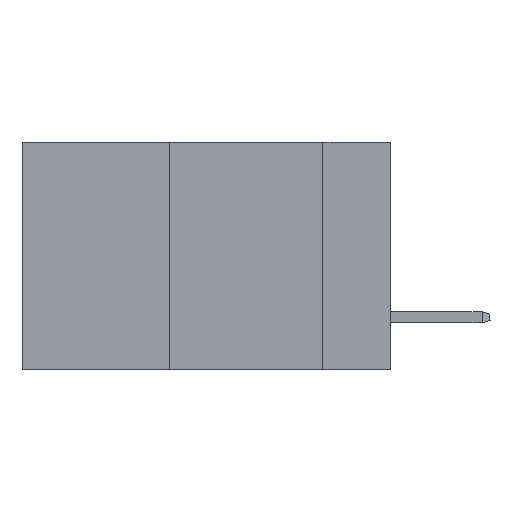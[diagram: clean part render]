
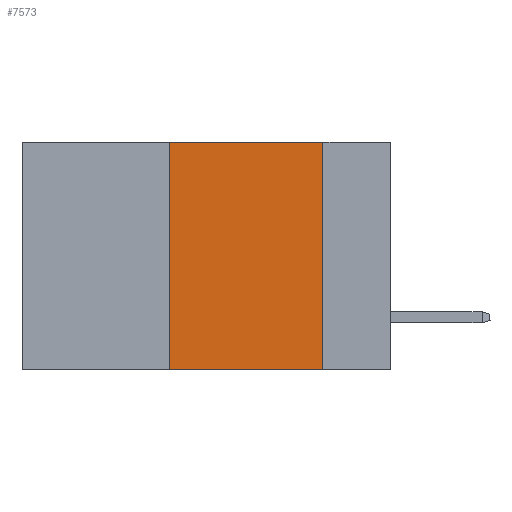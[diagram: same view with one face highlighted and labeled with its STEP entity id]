
A CAD part, left-side view. The second image highlights one B-rep face of the part: STEP entity #7573.
In plain terms, the highlighted planar face has unit normal (-1, 0, 0).
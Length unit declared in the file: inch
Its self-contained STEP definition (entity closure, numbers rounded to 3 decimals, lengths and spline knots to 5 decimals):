
#1581 = VERTEX_POINT ( 'NONE', #14168 ) ;
#2299 = CARTESIAN_POINT ( 'NONE',  ( 0., 0.6, 0. ) ) ;
#2630 = DIRECTION ( 'NONE',  ( 0., 0., 1. ) ) ;
#3294 = VECTOR ( 'NONE', #2630, 39.37008 ) ;
#3382 = CARTESIAN_POINT ( 'NONE',  ( 0., 0.36, -0.37 ) ) ;
#4561 = ORIENTED_EDGE ( 'NONE', *, *, #7499, .F. ) ;
#5371 = CARTESIAN_POINT ( 'NONE',  ( 0., 0.11, 0. ) ) ;
#6660 = EDGE_CURVE ( 'NONE', #1581, #9404, #7897, .T. ) ;
#7148 = ORIENTED_EDGE ( 'NONE', *, *, #10180, .F. ) ;
#7499 = EDGE_CURVE ( 'NONE', #10440, #1581, #23999, .T. ) ;
#7573 = ADVANCED_FACE ( 'NONE', ( #11313 ), #7975, .F. ) ;
#7605 = CARTESIAN_POINT ( 'NONE',  ( 0., 0.11, -0.37 ) ) ;
#7897 = LINE ( 'NONE', #5371, #25316 ) ;
#7975 = PLANE ( 'NONE',  #8375 ) ;
#8375 = AXIS2_PLACEMENT_3D ( 'NONE', #22219, #16552, #22559 ) ;
#8547 = EDGE_LOOP ( 'NONE', ( #12255, #4561, #7148, #10906 ) ) ;
#8952 = CARTESIAN_POINT ( 'NONE',  ( 0., 0.6, -0.37 ) ) ;
#9338 = CARTESIAN_POINT ( 'NONE',  ( 0., 0.36, 0. ) ) ;
#9404 = VERTEX_POINT ( 'NONE', #7605 ) ;
#10180 = EDGE_CURVE ( 'NONE', #14652, #10440, #14028, .T. ) ;
#10440 = VERTEX_POINT ( 'NONE', #9338 ) ;
#10906 = ORIENTED_EDGE ( 'NONE', *, *, #21439, .T. ) ;
#11313 = FACE_OUTER_BOUND ( 'NONE', #8547, .T. ) ;
#12255 = ORIENTED_EDGE ( 'NONE', *, *, #6660, .F. ) ;
#14028 = LINE ( 'NONE', #23514, #3294 ) ;
#14168 = CARTESIAN_POINT ( 'NONE',  ( 0., 0.11, 0. ) ) ;
#14652 = VERTEX_POINT ( 'NONE', #3382 ) ;
#15391 = LINE ( 'NONE', #8952, #19864 ) ;
#15756 = DIRECTION ( 'NONE',  ( 0., -1., 0. ) ) ;
#16365 = VECTOR ( 'NONE', #16475, 39.37008 ) ;
#16475 = DIRECTION ( 'NONE',  ( 0., -1., 0. ) ) ;
#16552 = DIRECTION ( 'NONE',  ( 1., 0., 0. ) ) ;
#19864 = VECTOR ( 'NONE', #15756, 39.37008 ) ;
#21439 = EDGE_CURVE ( 'NONE', #14652, #9404, #15391, .T. ) ;
#21597 = DIRECTION ( 'NONE',  ( 0., 0., -1. ) ) ;
#22219 = CARTESIAN_POINT ( 'NONE',  ( 0., 0.6, 0. ) ) ;
#22559 = DIRECTION ( 'NONE',  ( 0., 0., -1. ) ) ;
#23514 = CARTESIAN_POINT ( 'NONE',  ( 0., 0.36, 0. ) ) ;
#23999 = LINE ( 'NONE', #2299, #16365 ) ;
#25316 = VECTOR ( 'NONE', #21597, 39.37008 ) ;
